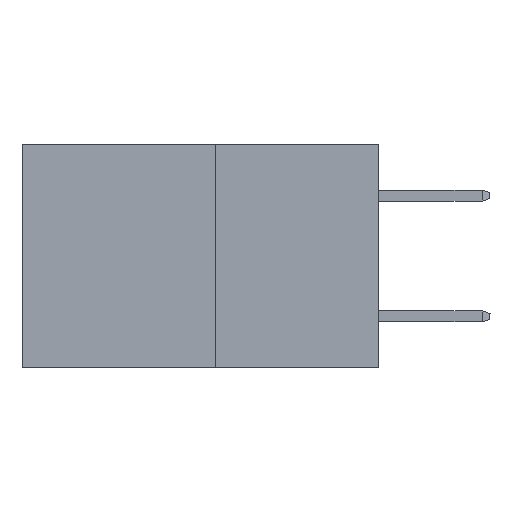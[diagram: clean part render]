
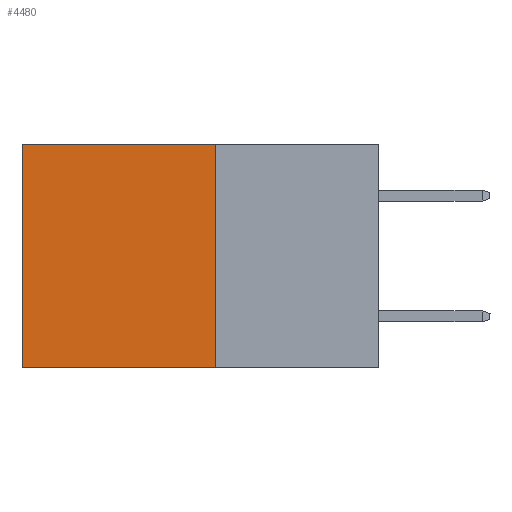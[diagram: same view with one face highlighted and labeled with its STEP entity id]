
A CAD part, left-side view. The second image highlights one B-rep face of the part: STEP entity #4480.
In plain terms, the highlighted planar face has unit normal (-1, 0, 0).
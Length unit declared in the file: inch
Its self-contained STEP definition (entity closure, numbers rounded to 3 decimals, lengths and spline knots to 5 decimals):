
#467 = CARTESIAN_POINT ( 'NONE',  ( 0.277, 0.27, 0. ) ) ;
#532 = DIRECTION ( 'NONE',  ( 0., 1., 0. ) ) ;
#928 = DIRECTION ( 'NONE',  ( 0., 1., 0. ) ) ;
#1523 = AXIS2_PLACEMENT_3D ( 'NONE', #5106, #7354, #10288 ) ;
#1640 = EDGE_LOOP ( 'NONE', ( #7246, #4573, #4446, #3251 ) ) ;
#1669 = VECTOR ( 'NONE', #532, 39.37008 ) ;
#1682 = DIRECTION ( 'NONE',  ( 0., 0., -1. ) ) ;
#1910 = VERTEX_POINT ( 'NONE', #467 ) ;
#2012 = VERTEX_POINT ( 'NONE', #11247 ) ;
#2190 = EDGE_CURVE ( 'NONE', #3488, #3309, #4441, .T. ) ;
#2580 = FACE_OUTER_BOUND ( 'NONE', #1640, .T. ) ;
#3251 = ORIENTED_EDGE ( 'NONE', *, *, #5912, .T. ) ;
#3309 = VERTEX_POINT ( 'NONE', #4071 ) ;
#3488 = VERTEX_POINT ( 'NONE', #10700 ) ;
#4071 = CARTESIAN_POINT ( 'NONE',  ( 0.277, 0.59, -0.37 ) ) ;
#4441 = LINE ( 'NONE', #6014, #8833 ) ;
#4446 = ORIENTED_EDGE ( 'NONE', *, *, #5645, .F. ) ;
#4480 = ADVANCED_FACE ( 'NONE', ( #2580 ), #8597, .F. ) ;
#4573 = ORIENTED_EDGE ( 'NONE', *, *, #4977, .F. ) ;
#4977 = EDGE_CURVE ( 'NONE', #2012, #3309, #11347, .T. ) ;
#5106 = CARTESIAN_POINT ( 'NONE',  ( 0.277, 0.27, -0.37 ) ) ;
#5645 = EDGE_CURVE ( 'NONE', #1910, #2012, #6783, .T. ) ;
#5912 = EDGE_CURVE ( 'NONE', #1910, #3488, #6654, .T. ) ;
#6014 = CARTESIAN_POINT ( 'NONE',  ( 0.277, 0.59, -0.37 ) ) ;
#6370 = DIRECTION ( 'NONE',  ( 0., 0., -1. ) ) ;
#6654 = LINE ( 'NONE', #9280, #1669 ) ;
#6783 = LINE ( 'NONE', #9335, #8774 ) ;
#7246 = ORIENTED_EDGE ( 'NONE', *, *, #2190, .T. ) ;
#7354 = DIRECTION ( 'NONE',  ( 1., 0., 0. ) ) ;
#8597 = PLANE ( 'NONE',  #1523 ) ;
#8774 = VECTOR ( 'NONE', #1682, 39.37008 ) ;
#8833 = VECTOR ( 'NONE', #6370, 39.37008 ) ;
#9280 = CARTESIAN_POINT ( 'NONE',  ( 0.277, 0.27, 0. ) ) ;
#9335 = CARTESIAN_POINT ( 'NONE',  ( 0.277, 0.27, -0.37 ) ) ;
#10288 = DIRECTION ( 'NONE',  ( 0., 0., -1. ) ) ;
#10700 = CARTESIAN_POINT ( 'NONE',  ( 0.277, 0.59, 0. ) ) ;
#11084 = CARTESIAN_POINT ( 'NONE',  ( 0.277, 0.27, -0.37 ) ) ;
#11102 = VECTOR ( 'NONE', #928, 39.37008 ) ;
#11247 = CARTESIAN_POINT ( 'NONE',  ( 0.277, 0.27, -0.37 ) ) ;
#11347 = LINE ( 'NONE', #11084, #11102 ) ;
